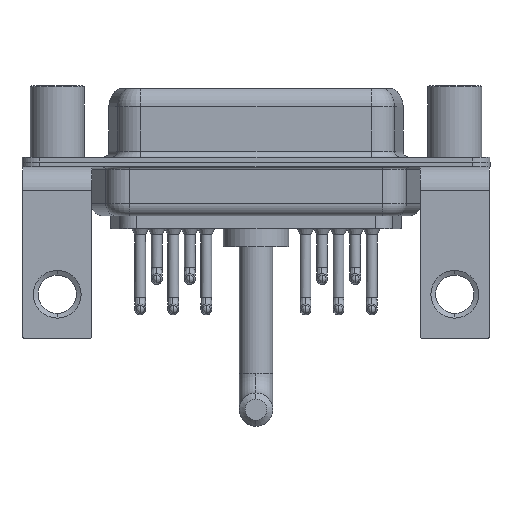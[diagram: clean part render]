
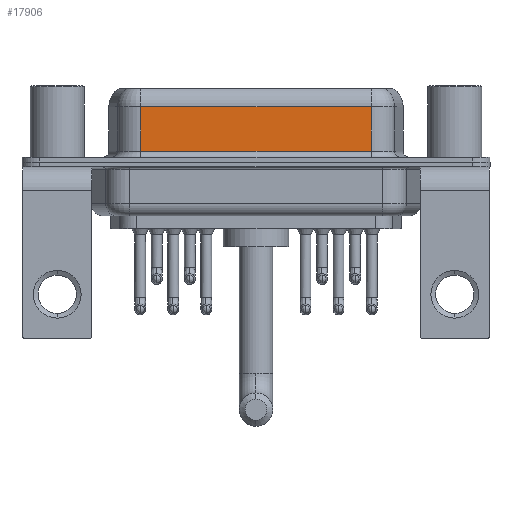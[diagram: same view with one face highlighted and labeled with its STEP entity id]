
A CAD part, front view. The second image highlights one B-rep face of the part: STEP entity #17906.
In plain terms, the highlighted planar face has unit normal (0, -1, 0).
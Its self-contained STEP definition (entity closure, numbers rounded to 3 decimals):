
#280 = DIRECTION ( 'NONE',  ( 0., 0., -1. ) ) ;
#707 = LINE ( 'NONE', #19884, #2950 ) ;
#1228 = CARTESIAN_POINT ( 'NONE',  ( 26.287, -3.95, 4.65 ) ) ;
#1507 = ORIENTED_EDGE ( 'NONE', *, *, #13866, .T. ) ;
#2795 = VERTEX_POINT ( 'NONE', #9328 ) ;
#2950 = VECTOR ( 'NONE', #280, 1000. ) ;
#5175 = EDGE_LOOP ( 'NONE', ( #20804, #1507, #17126, #16254 ) ) ;
#6321 = LINE ( 'NONE', #19375, #19139 ) ;
#6453 = PLANE ( 'NONE',  #15710 ) ;
#6659 = EDGE_CURVE ( 'NONE', #14756, #15169, #15126, .T. ) ;
#6967 = EDGE_CURVE ( 'NONE', #19243, #15169, #6321, .T. ) ;
#9079 = LINE ( 'NONE', #1228, #14851 ) ;
#9328 = CARTESIAN_POINT ( 'NONE',  ( 7.013, -3.95, 4.65 ) ) ;
#10777 = CARTESIAN_POINT ( 'NONE',  ( 7.013, -3.95, 0.9 ) ) ;
#11163 = FACE_OUTER_BOUND ( 'NONE', #5175, .T. ) ;
#12650 = DIRECTION ( 'NONE',  ( 1., 0., 0. ) ) ;
#13005 = DIRECTION ( 'NONE',  ( 0., 1., 0. ) ) ;
#13688 = VECTOR ( 'NONE', #19830, 1000. ) ;
#13866 = EDGE_CURVE ( 'NONE', #14756, #2795, #9079, .T. ) ;
#14136 = DIRECTION ( 'NONE',  ( -1., 0., 0. ) ) ;
#14756 = VERTEX_POINT ( 'NONE', #17488 ) ;
#14851 = VECTOR ( 'NONE', #14136, 1000. ) ;
#15126 = LINE ( 'NONE', #19719, #13688 ) ;
#15169 = VERTEX_POINT ( 'NONE', #19825 ) ;
#15710 = AXIS2_PLACEMENT_3D ( 'NONE', #20924, #13005, #17596 ) ;
#16254 = ORIENTED_EDGE ( 'NONE', *, *, #6967, .T. ) ;
#17126 = ORIENTED_EDGE ( 'NONE', *, *, #18410, .T. ) ;
#17488 = CARTESIAN_POINT ( 'NONE',  ( 26.287, -3.95, 4.65 ) ) ;
#17596 = DIRECTION ( 'NONE',  ( 0., 0., 1. ) ) ;
#17906 = ADVANCED_FACE ( 'NONE', ( #11163 ), #6453, .F. ) ;
#18410 = EDGE_CURVE ( 'NONE', #2795, #19243, #707, .T. ) ;
#19139 = VECTOR ( 'NONE', #12650, 1000. ) ;
#19243 = VERTEX_POINT ( 'NONE', #10777 ) ;
#19375 = CARTESIAN_POINT ( 'NONE',  ( 26.287, -3.95, 0.9 ) ) ;
#19719 = CARTESIAN_POINT ( 'NONE',  ( 26.287, -3.95, 6.4 ) ) ;
#19825 = CARTESIAN_POINT ( 'NONE',  ( 26.287, -3.95, 0.9 ) ) ;
#19830 = DIRECTION ( 'NONE',  ( 0., 0., -1. ) ) ;
#19884 = CARTESIAN_POINT ( 'NONE',  ( 7.013, -3.95, 6.4 ) ) ;
#20804 = ORIENTED_EDGE ( 'NONE', *, *, #6659, .F. ) ;
#20924 = CARTESIAN_POINT ( 'NONE',  ( 26.287, -3.95, 6.4 ) ) ;
